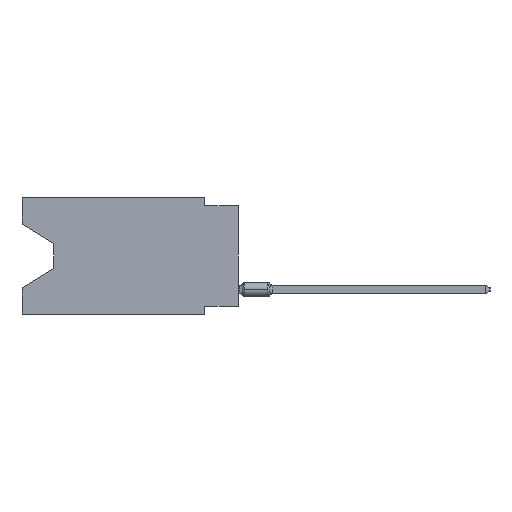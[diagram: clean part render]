
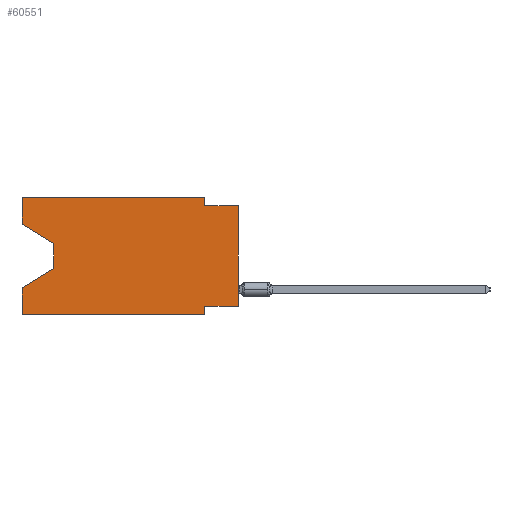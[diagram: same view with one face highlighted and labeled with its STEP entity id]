
A CAD part, left-side view. The second image highlights one B-rep face of the part: STEP entity #60551.
In plain terms, the highlighted planar face has unit normal (-1, 0, 0).
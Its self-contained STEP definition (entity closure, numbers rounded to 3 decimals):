
#212 = EDGE_CURVE ( 'NONE', #13070, #55817, #55947, .T. ) ;
#247 = EDGE_CURVE ( 'NONE', #39532, #22010, #6975, .T. ) ;
#1255 = VERTEX_POINT ( 'NONE', #57386 ) ;
#1446 = DIRECTION ( 'NONE',  ( 0., 0., 1. ) ) ;
#1556 = CARTESIAN_POINT ( 'NONE',  ( 0., 0., 0. ) ) ;
#1798 = CARTESIAN_POINT ( 'NONE',  ( 0., 16.383, 0. ) ) ;
#1865 = DIRECTION ( 'NONE',  ( 0., -0.855, -0.519 ) ) ;
#2501 = LINE ( 'NONE', #1556, #63604 ) ;
#3506 = VERTEX_POINT ( 'NONE', #11638 ) ;
#3750 = CARTESIAN_POINT ( 'NONE',  ( 0., 16.383, 0. ) ) ;
#3995 = EDGE_CURVE ( 'NONE', #13070, #6112, #32421, .T. ) ;
#6112 = VERTEX_POINT ( 'NONE', #59967 ) ;
#6975 = LINE ( 'NONE', #26870, #49682 ) ;
#7517 = CARTESIAN_POINT ( 'NONE',  ( 0., 0., -8.255 ) ) ;
#9475 = EDGE_CURVE ( 'NONE', #1255, #51187, #24051, .T. ) ;
#10663 = EDGE_CURVE ( 'NONE', #3506, #39532, #19612, .T. ) ;
#11638 = CARTESIAN_POINT ( 'NONE',  ( 0., 2.54, 0. ) ) ;
#11902 = VERTEX_POINT ( 'NONE', #41153 ) ;
#12010 = AXIS2_PLACEMENT_3D ( 'NONE', #50815, #56660, #26948 ) ;
#13045 = ORIENTED_EDGE ( 'NONE', *, *, #38427, .F. ) ;
#13070 = VERTEX_POINT ( 'NONE', #21700 ) ;
#13097 = EDGE_CURVE ( 'NONE', #11902, #27202, #55987, .T. ) ;
#13307 = CARTESIAN_POINT ( 'NONE',  ( 0., 13.97, -3.505 ) ) ;
#14220 = LINE ( 'NONE', #24000, #20143 ) ;
#16472 = CARTESIAN_POINT ( 'NONE',  ( 0., 2.54, -8.89 ) ) ;
#18375 = DIRECTION ( 'NONE',  ( 0., -1., 0. ) ) ;
#18725 = CARTESIAN_POINT ( 'NONE',  ( 0., 16.383, -6.852 ) ) ;
#19489 = VECTOR ( 'NONE', #1446, 1000. ) ;
#19612 = LINE ( 'NONE', #29737, #36945 ) ;
#20143 = VECTOR ( 'NONE', #63489, 1000. ) ;
#20614 = ORIENTED_EDGE ( 'NONE', *, *, #41601, .F. ) ;
#21700 = CARTESIAN_POINT ( 'NONE',  ( 0., 16.383, -8.89 ) ) ;
#22010 = VERTEX_POINT ( 'NONE', #42982 ) ;
#22380 = PLANE ( 'NONE',  #12010 ) ;
#22998 = ORIENTED_EDGE ( 'NONE', *, *, #10663, .F. ) ;
#24000 = CARTESIAN_POINT ( 'NONE',  ( 0., 13.97, -5.385 ) ) ;
#24051 = LINE ( 'NONE', #13307, #61777 ) ;
#26870 = CARTESIAN_POINT ( 'NONE',  ( 0., 0., -0.635 ) ) ;
#26891 = DIRECTION ( 'NONE',  ( 0., 0., -1. ) ) ;
#26927 = ORIENTED_EDGE ( 'NONE', *, *, #13097, .F. ) ;
#26948 = DIRECTION ( 'NONE',  ( 0., 0., -1. ) ) ;
#27202 = VERTEX_POINT ( 'NONE', #63500 ) ;
#27464 = VECTOR ( 'NONE', #54631, 1000. ) ;
#28609 = VERTEX_POINT ( 'NONE', #61339 ) ;
#28852 = LINE ( 'NONE', #58866, #27464 ) ;
#28949 = EDGE_CURVE ( 'NONE', #11902, #1255, #61579, .T. ) ;
#29737 = CARTESIAN_POINT ( 'NONE',  ( 0., 2.54, 0. ) ) ;
#30966 = VECTOR ( 'NONE', #55669, 1000. ) ;
#31076 = EDGE_CURVE ( 'NONE', #51187, #55817, #14220, .T. ) ;
#32189 = VECTOR ( 'NONE', #18375, 1000. ) ;
#32421 = LINE ( 'NONE', #57871, #32189 ) ;
#33955 = ORIENTED_EDGE ( 'NONE', *, *, #3995, .T. ) ;
#34436 = ORIENTED_EDGE ( 'NONE', *, *, #31076, .T. ) ;
#36770 = DIRECTION ( 'NONE',  ( 0., 0., 1. ) ) ;
#36945 = VECTOR ( 'NONE', #39520, 1000. ) ;
#38427 = EDGE_CURVE ( 'NONE', #27202, #3506, #43885, .T. ) ;
#38553 = VECTOR ( 'NONE', #26891, 1000. ) ;
#39520 = DIRECTION ( 'NONE',  ( 0., 0., -1. ) ) ;
#39532 = VERTEX_POINT ( 'NONE', #48153 ) ;
#40723 = CARTESIAN_POINT ( 'NONE',  ( 0., 16.383, -2.038 ) ) ;
#41153 = CARTESIAN_POINT ( 'NONE',  ( 0., 16.383, -2.038 ) ) ;
#41601 = EDGE_CURVE ( 'NONE', #28609, #6112, #60552, .T. ) ;
#42982 = CARTESIAN_POINT ( 'NONE',  ( 0., 0., -0.635 ) ) ;
#43885 = LINE ( 'NONE', #3750, #62468 ) ;
#43978 = DIRECTION ( 'NONE',  ( 0., 0., -1. ) ) ;
#44402 = EDGE_CURVE ( 'NONE', #58970, #22010, #2501, .T. ) ;
#44518 = ORIENTED_EDGE ( 'NONE', *, *, #212, .F. ) ;
#44852 = DIRECTION ( 'NONE',  ( 0., -1., 0. ) ) ;
#46159 = CARTESIAN_POINT ( 'NONE',  ( 0., 16.383, 0. ) ) ;
#46192 = EDGE_LOOP ( 'NONE', ( #57314, #48944, #34436, #44518, #33955, #20614, #61146, #47088, #46933, #22998, #13045, #26927 ) ) ;
#46792 = DIRECTION ( 'NONE',  ( 0., -1., 0. ) ) ;
#46933 = ORIENTED_EDGE ( 'NONE', *, *, #247, .F. ) ;
#47088 = ORIENTED_EDGE ( 'NONE', *, *, #44402, .T. ) ;
#48153 = CARTESIAN_POINT ( 'NONE',  ( 0., 2.54, -0.635 ) ) ;
#48944 = ORIENTED_EDGE ( 'NONE', *, *, #9475, .T. ) ;
#49682 = VECTOR ( 'NONE', #46792, 1000. ) ;
#50815 = CARTESIAN_POINT ( 'NONE',  ( 0., 16.383, 0. ) ) ;
#51187 = VERTEX_POINT ( 'NONE', #59064 ) ;
#54372 = VECTOR ( 'NONE', #1865, 1000. ) ;
#54631 = DIRECTION ( 'NONE',  ( 0., 1., 0. ) ) ;
#55669 = DIRECTION ( 'NONE',  ( 0., 0., 1. ) ) ;
#55817 = VERTEX_POINT ( 'NONE', #18725 ) ;
#55947 = LINE ( 'NONE', #46159, #19489 ) ;
#55987 = LINE ( 'NONE', #1798, #30966 ) ;
#56028 = FACE_OUTER_BOUND ( 'NONE', #46192, .T. ) ;
#56660 = DIRECTION ( 'NONE',  ( 1., 0., 0. ) ) ;
#57135 = EDGE_CURVE ( 'NONE', #58970, #28609, #28852, .T. ) ;
#57314 = ORIENTED_EDGE ( 'NONE', *, *, #28949, .T. ) ;
#57386 = CARTESIAN_POINT ( 'NONE',  ( 0., 13.97, -3.505 ) ) ;
#57871 = CARTESIAN_POINT ( 'NONE',  ( 0., 16.383, -8.89 ) ) ;
#58866 = CARTESIAN_POINT ( 'NONE',  ( 0., 0., -8.255 ) ) ;
#58970 = VERTEX_POINT ( 'NONE', #7517 ) ;
#59064 = CARTESIAN_POINT ( 'NONE',  ( 0., 13.97, -5.385 ) ) ;
#59967 = CARTESIAN_POINT ( 'NONE',  ( 0., 2.54, -8.89 ) ) ;
#60551 = ADVANCED_FACE ( 'NONE', ( #56028 ), #22380, .F. ) ;
#60552 = LINE ( 'NONE', #16472, #38553 ) ;
#61146 = ORIENTED_EDGE ( 'NONE', *, *, #57135, .F. ) ;
#61339 = CARTESIAN_POINT ( 'NONE',  ( 0., 2.54, -8.255 ) ) ;
#61579 = LINE ( 'NONE', #40723, #54372 ) ;
#61777 = VECTOR ( 'NONE', #43978, 1000. ) ;
#62468 = VECTOR ( 'NONE', #44852, 1000. ) ;
#63489 = DIRECTION ( 'NONE',  ( 0., 0.855, -0.519 ) ) ;
#63500 = CARTESIAN_POINT ( 'NONE',  ( 0., 16.383, 0. ) ) ;
#63604 = VECTOR ( 'NONE', #36770, 1000. ) ;
